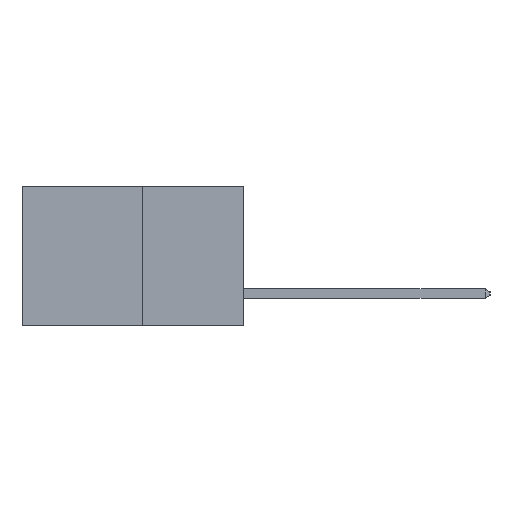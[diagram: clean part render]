
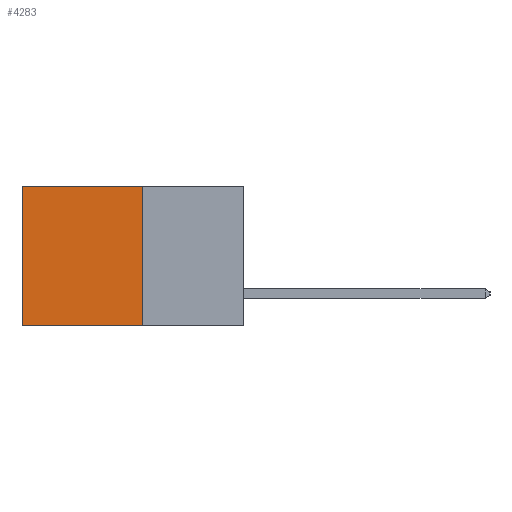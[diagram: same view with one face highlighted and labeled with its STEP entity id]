
A CAD part, left-side view. The second image highlights one B-rep face of the part: STEP entity #4283.
In plain terms, the highlighted planar face has unit normal (-1, 0, 0).
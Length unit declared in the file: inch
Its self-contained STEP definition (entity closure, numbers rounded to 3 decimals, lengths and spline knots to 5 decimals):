
#567 = EDGE_CURVE ( 'NONE', #4103, #5740, #5408, .T. ) ;
#703 = FACE_OUTER_BOUND ( 'NONE', #2496, .T. ) ;
#905 = EDGE_CURVE ( 'NONE', #1714, #4062, #2049, .T. ) ;
#1110 = LINE ( 'NONE', #1563, #2418 ) ;
#1170 = PLANE ( 'NONE',  #4963 ) ;
#1316 = ORIENTED_EDGE ( 'NONE', *, *, #905, .T. ) ;
#1563 = CARTESIAN_POINT ( 'NONE',  ( 0.277, 0.59, -0.37 ) ) ;
#1597 = EDGE_CURVE ( 'NONE', #1714, #4103, #7980, .T. ) ;
#1700 = CARTESIAN_POINT ( 'NONE',  ( 0.277, 0.59, 0. ) ) ;
#1714 = VERTEX_POINT ( 'NONE', #8844 ) ;
#1950 = DIRECTION ( 'NONE',  ( 1., 0., 0. ) ) ;
#2049 = LINE ( 'NONE', #9241, #7869 ) ;
#2327 = DIRECTION ( 'NONE',  ( 0., 0., -1. ) ) ;
#2418 = VECTOR ( 'NONE', #2327, 39.37008 ) ;
#2496 = EDGE_LOOP ( 'NONE', ( #9801, #8699, #5653, #1316 ) ) ;
#3637 = EDGE_CURVE ( 'NONE', #4062, #5740, #1110, .T. ) ;
#4062 = VERTEX_POINT ( 'NONE', #1700 ) ;
#4103 = VERTEX_POINT ( 'NONE', #7114 ) ;
#4283 = ADVANCED_FACE ( 'NONE', ( #703 ), #1170, .F. ) ;
#4854 = CARTESIAN_POINT ( 'NONE',  ( 0.277, 0.59, -0.37 ) ) ;
#4963 = AXIS2_PLACEMENT_3D ( 'NONE', #6567, #1950, #7307 ) ;
#5408 = LINE ( 'NONE', #9158, #7440 ) ;
#5653 = ORIENTED_EDGE ( 'NONE', *, *, #1597, .F. ) ;
#5740 = VERTEX_POINT ( 'NONE', #4854 ) ;
#6567 = CARTESIAN_POINT ( 'NONE',  ( 0.277, 0.27, -0.37 ) ) ;
#6786 = DIRECTION ( 'NONE',  ( 0., 0., -1. ) ) ;
#7114 = CARTESIAN_POINT ( 'NONE',  ( 0.277, 0.27, -0.37 ) ) ;
#7280 = DIRECTION ( 'NONE',  ( 0., 1., 0. ) ) ;
#7307 = DIRECTION ( 'NONE',  ( 0., 0., -1. ) ) ;
#7440 = VECTOR ( 'NONE', #7535, 39.37008 ) ;
#7535 = DIRECTION ( 'NONE',  ( 0., 1., 0. ) ) ;
#7869 = VECTOR ( 'NONE', #7280, 39.37008 ) ;
#7980 = LINE ( 'NONE', #8755, #9718 ) ;
#8699 = ORIENTED_EDGE ( 'NONE', *, *, #567, .F. ) ;
#8755 = CARTESIAN_POINT ( 'NONE',  ( 0.277, 0.27, -0.37 ) ) ;
#8844 = CARTESIAN_POINT ( 'NONE',  ( 0.277, 0.27, 0. ) ) ;
#9158 = CARTESIAN_POINT ( 'NONE',  ( 0.277, 0.27, -0.37 ) ) ;
#9241 = CARTESIAN_POINT ( 'NONE',  ( 0.277, 0.27, 0. ) ) ;
#9718 = VECTOR ( 'NONE', #6786, 39.37008 ) ;
#9801 = ORIENTED_EDGE ( 'NONE', *, *, #3637, .T. ) ;
